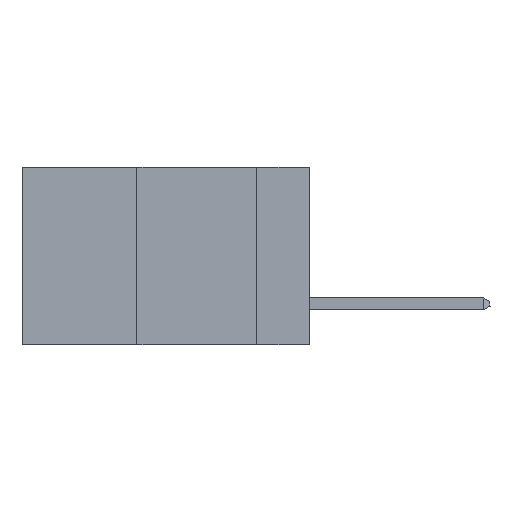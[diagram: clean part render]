
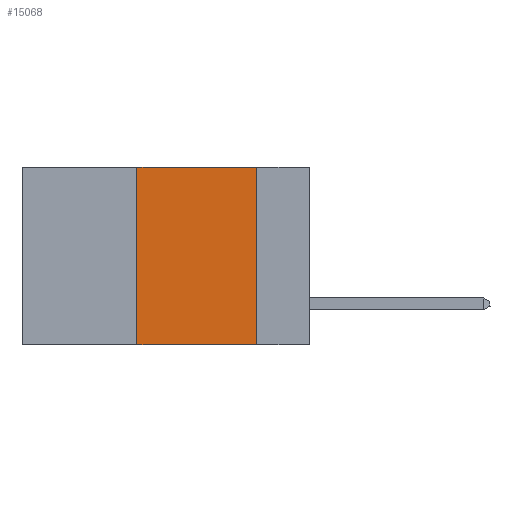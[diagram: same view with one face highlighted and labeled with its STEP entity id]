
A CAD part, left-side view. The second image highlights one B-rep face of the part: STEP entity #15068.
In plain terms, the highlighted planar face has unit normal (-1, 0, 0).
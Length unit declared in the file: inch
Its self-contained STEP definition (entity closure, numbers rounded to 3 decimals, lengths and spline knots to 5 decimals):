
#253 = DIRECTION ( 'NONE',  ( 0., 0., -1. ) ) ;
#263 = AXIS2_PLACEMENT_3D ( 'NONE', #5332, #13651, #253 ) ;
#807 = CARTESIAN_POINT ( 'NONE',  ( 0., 0.11, 0. ) ) ;
#1089 = EDGE_CURVE ( 'NONE', #20587, #1112, #12522, .T. ) ;
#1112 = VERTEX_POINT ( 'NONE', #19249 ) ;
#1309 = CARTESIAN_POINT ( 'NONE',  ( 0., 0.36, 0. ) ) ;
#1494 = CARTESIAN_POINT ( 'NONE',  ( 0., 0.6, -0.37 ) ) ;
#1507 = VECTOR ( 'NONE', #19702, 39.37008 ) ;
#1560 = LINE ( 'NONE', #12519, #4405 ) ;
#2647 = FACE_OUTER_BOUND ( 'NONE', #20877, .T. ) ;
#3447 = CARTESIAN_POINT ( 'NONE',  ( 0., 0.36, -0.37 ) ) ;
#4405 = VECTOR ( 'NONE', #7311, 39.37008 ) ;
#4699 = EDGE_CURVE ( 'NONE', #14799, #20587, #1560, .T. ) ;
#5254 = PLANE ( 'NONE',  #263 ) ;
#5332 = CARTESIAN_POINT ( 'NONE',  ( 0., 0.6, 0. ) ) ;
#5840 = VERTEX_POINT ( 'NONE', #3447 ) ;
#6788 = ORIENTED_EDGE ( 'NONE', *, *, #4699, .F. ) ;
#7175 = EDGE_CURVE ( 'NONE', #5840, #1112, #19619, .T. ) ;
#7311 = DIRECTION ( 'NONE',  ( 0., -1., 0. ) ) ;
#12519 = CARTESIAN_POINT ( 'NONE',  ( 0., 0.6, 0. ) ) ;
#12522 = LINE ( 'NONE', #807, #18641 ) ;
#12801 = CARTESIAN_POINT ( 'NONE',  ( 0., 0.36, 0. ) ) ;
#13303 = CARTESIAN_POINT ( 'NONE',  ( 0., 0.11, 0. ) ) ;
#13651 = DIRECTION ( 'NONE',  ( 1., 0., 0. ) ) ;
#13984 = ORIENTED_EDGE ( 'NONE', *, *, #17940, .F. ) ;
#14799 = VERTEX_POINT ( 'NONE', #1309 ) ;
#15068 = ADVANCED_FACE ( 'NONE', ( #2647 ), #5254, .F. ) ;
#15227 = ORIENTED_EDGE ( 'NONE', *, *, #7175, .T. ) ;
#15942 = DIRECTION ( 'NONE',  ( 0., 0., -1. ) ) ;
#17235 = VECTOR ( 'NONE', #21511, 39.37008 ) ;
#17940 = EDGE_CURVE ( 'NONE', #5840, #14799, #20727, .T. ) ;
#18641 = VECTOR ( 'NONE', #15942, 39.37008 ) ;
#19249 = CARTESIAN_POINT ( 'NONE',  ( 0., 0.11, -0.37 ) ) ;
#19619 = LINE ( 'NONE', #1494, #17235 ) ;
#19702 = DIRECTION ( 'NONE',  ( 0., 0., 1. ) ) ;
#20126 = ORIENTED_EDGE ( 'NONE', *, *, #1089, .F. ) ;
#20587 = VERTEX_POINT ( 'NONE', #13303 ) ;
#20727 = LINE ( 'NONE', #12801, #1507 ) ;
#20877 = EDGE_LOOP ( 'NONE', ( #20126, #6788, #13984, #15227 ) ) ;
#21511 = DIRECTION ( 'NONE',  ( 0., -1., 0. ) ) ;
